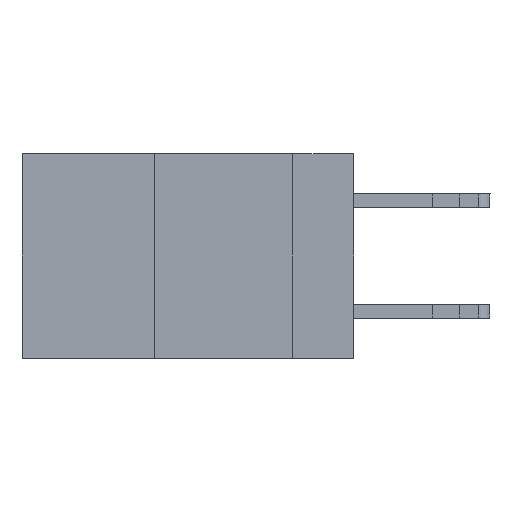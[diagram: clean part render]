
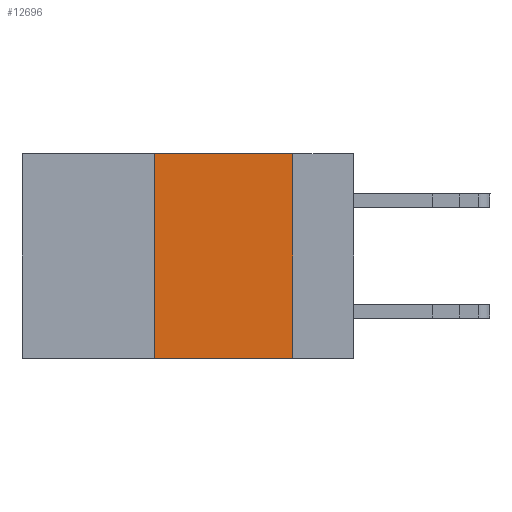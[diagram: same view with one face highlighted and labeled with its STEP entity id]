
A CAD part, left-side view. The second image highlights one B-rep face of the part: STEP entity #12696.
In plain terms, the highlighted planar face has unit normal (-1, 0, 0).
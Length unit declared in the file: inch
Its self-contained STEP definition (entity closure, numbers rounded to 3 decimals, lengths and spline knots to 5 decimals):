
#97 = VERTEX_POINT ( 'NONE', #17275 ) ;
#102 = FACE_OUTER_BOUND ( 'NONE', #8687, .T. ) ;
#151 = CARTESIAN_POINT ( 'NONE',  ( 0., 0.11, -0.37 ) ) ;
#812 = VECTOR ( 'NONE', #9123, 39.37008 ) ;
#994 = VERTEX_POINT ( 'NONE', #151 ) ;
#1665 = CARTESIAN_POINT ( 'NONE',  ( 0., 0.6, -0.37 ) ) ;
#1752 = ORIENTED_EDGE ( 'NONE', *, *, #9529, .F. ) ;
#2131 = VECTOR ( 'NONE', #6663, 39.37008 ) ;
#2252 = LINE ( 'NONE', #4985, #812 ) ;
#2935 = ORIENTED_EDGE ( 'NONE', *, *, #17759, .F. ) ;
#3089 = DIRECTION ( 'NONE',  ( 0., -1., 0. ) ) ;
#4985 = CARTESIAN_POINT ( 'NONE',  ( 0., 0.6, 0. ) ) ;
#5804 = DIRECTION ( 'NONE',  ( 0., 0., -1. ) ) ;
#5810 = VERTEX_POINT ( 'NONE', #18029 ) ;
#6465 = EDGE_CURVE ( 'NONE', #5810, #994, #16201, .T. ) ;
#6663 = DIRECTION ( 'NONE',  ( 0., 0., 1. ) ) ;
#7378 = ORIENTED_EDGE ( 'NONE', *, *, #12492, .F. ) ;
#7911 = CARTESIAN_POINT ( 'NONE',  ( 0., 0.36, 0. ) ) ;
#8247 = VERTEX_POINT ( 'NONE', #13416 ) ;
#8663 = AXIS2_PLACEMENT_3D ( 'NONE', #17344, #11636, #5804 ) ;
#8687 = EDGE_LOOP ( 'NONE', ( #7378, #1752, #2935, #13446 ) ) ;
#9123 = DIRECTION ( 'NONE',  ( 0., -1., 0. ) ) ;
#9529 = EDGE_CURVE ( 'NONE', #8247, #97, #2252, .T. ) ;
#11076 = CARTESIAN_POINT ( 'NONE',  ( 0., 0.11, 0. ) ) ;
#11636 = DIRECTION ( 'NONE',  ( 1., 0., 0. ) ) ;
#12492 = EDGE_CURVE ( 'NONE', #97, #994, #18365, .T. ) ;
#12696 = ADVANCED_FACE ( 'NONE', ( #102 ), #14518, .F. ) ;
#12718 = VECTOR ( 'NONE', #3089, 39.37008 ) ;
#13416 = CARTESIAN_POINT ( 'NONE',  ( 0., 0.36, 0. ) ) ;
#13446 = ORIENTED_EDGE ( 'NONE', *, *, #6465, .T. ) ;
#14518 = PLANE ( 'NONE',  #8663 ) ;
#15200 = LINE ( 'NONE', #7911, #2131 ) ;
#16201 = LINE ( 'NONE', #1665, #12718 ) ;
#16409 = VECTOR ( 'NONE', #18275, 39.37008 ) ;
#17275 = CARTESIAN_POINT ( 'NONE',  ( 0., 0.11, 0. ) ) ;
#17344 = CARTESIAN_POINT ( 'NONE',  ( 0., 0.6, 0. ) ) ;
#17759 = EDGE_CURVE ( 'NONE', #5810, #8247, #15200, .T. ) ;
#18029 = CARTESIAN_POINT ( 'NONE',  ( 0., 0.36, -0.37 ) ) ;
#18275 = DIRECTION ( 'NONE',  ( 0., 0., -1. ) ) ;
#18365 = LINE ( 'NONE', #11076, #16409 ) ;
